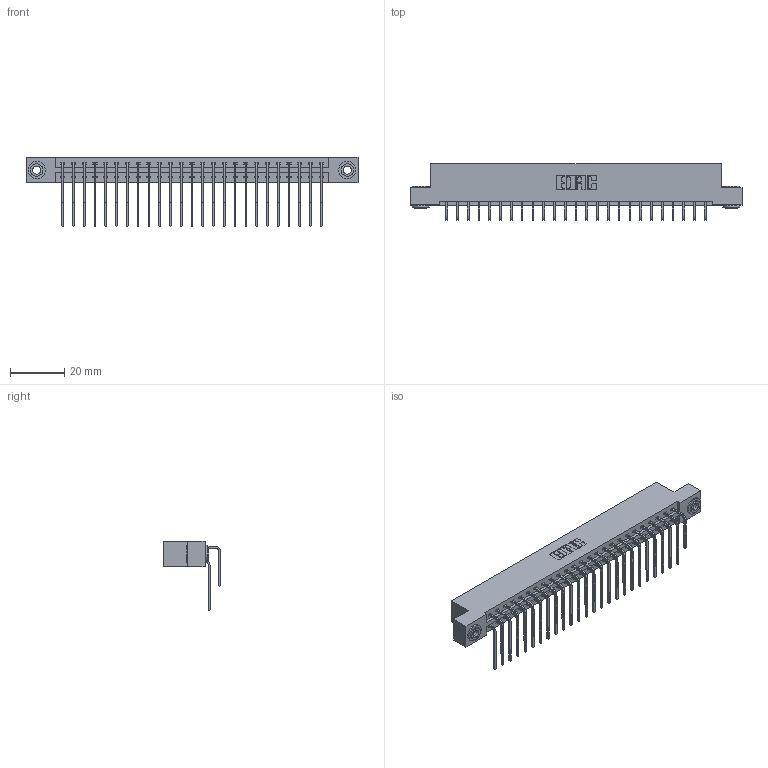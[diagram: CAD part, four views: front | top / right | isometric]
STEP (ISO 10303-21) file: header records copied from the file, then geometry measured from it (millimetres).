
FILE_DESCRIPTION (( 'STEP AP203' ), '1' );
FILE_NAME ('337-050-559-203.STEP', '2018-08-09T21:45:22', ( '' ), ( '' ), 'SwSTEP 2.0', 'SolidWorks 2016', '' );
FILE_SCHEMA (( 'CONFIG_CONTROL_DESIGN' ));
Length unit declared in the file: inch
Products named in the file (5): 337 Part_Flush Mounting Lugs - 0.156 Dia-TH; 345-292-001_558 559 Tail - 1; 345-292-001_559 Tail - 2; 345-250-002_345-250-002-102; 337-050-559-203
Assembly tree (53 placements, depth 2):
  337-050-559-203
    337 Part_Flush Mounting Lugs - 0.156 Dia-TH
    345-292-001_558 559 Tail - 1  x25
    345-292-001_559 Tail - 2  x25
    345-250-002_345-250-002-102  x2
Bounding box: 122.07 x 20.9 x 25.53 mm (x, y, z)
Volume: 12946.5 mm3; surface area: 16143.6 mm2
Topology: 53 solids, 53 shells, 2952 faces, 8737 edges, 5754 vertices
Faces by surface type: plane 2080, cylinder 864, cone 8
Entity records: 24016 total; most frequent: CARTESIAN_POINT 4080, ORIENTED_EDGE 3958, DIRECTION 3517, EDGE_CURVE 1979, LINE 1787, VECTOR 1787, VERTEX_POINT 1314, AXIS2_PLACEMENT_3D 865
